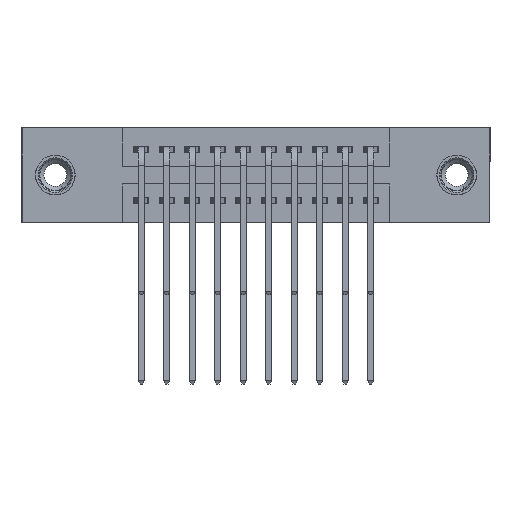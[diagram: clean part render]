
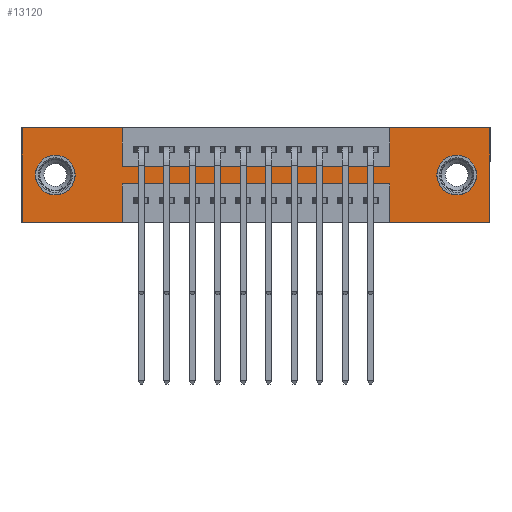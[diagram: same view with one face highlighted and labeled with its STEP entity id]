
A CAD part, front view. The second image highlights one B-rep face of the part: STEP entity #13120.
In plain terms, the highlighted planar face has unit normal (0, -1, 0).
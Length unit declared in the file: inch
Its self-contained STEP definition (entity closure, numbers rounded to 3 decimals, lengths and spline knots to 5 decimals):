
#68 = CARTESIAN_POINT ( 'NONE',  ( 0., 0., 0. ) ) ;
#136 = ORIENTED_EDGE ( 'NONE', *, *, #16094, .T. ) ;
#156 = VERTEX_POINT ( 'NONE', #68 ) ;
#206 = VECTOR ( 'NONE', #12975, 39.37008 ) ;
#285 = EDGE_CURVE ( 'NONE', #2101, #18559, #1158, .T. ) ;
#349 = CIRCLE ( 'NONE', #11111, 0.078 ) ;
#568 = CIRCLE ( 'NONE', #17081, 0.078 ) ;
#996 = CARTESIAN_POINT ( 'NONE',  ( 0.3925, 0., 0. ) ) ;
#1064 = EDGE_CURVE ( 'NONE', #9952, #18143, #1896, .T. ) ;
#1158 = LINE ( 'NONE', #2528, #15982 ) ;
#1196 = LINE ( 'NONE', #4455, #206 ) ;
#1268 = DIRECTION ( 'NONE',  ( 0., 0., 1. ) ) ;
#1285 = DIRECTION ( 'NONE',  ( 0., 0., -1. ) ) ;
#1363 = EDGE_LOOP ( 'NONE', ( #17937, #3118, #13664, #9716, #18570, #9848, #4302, #9397, #8794, #7609, #13158, #6612 ) ) ;
#1620 = FACE_BOUND ( 'NONE', #12168, .T. ) ;
#1694 = EDGE_CURVE ( 'NONE', #12277, #9224, #8646, .T. ) ;
#1896 = CIRCLE ( 'NONE', #10928, 0.078 ) ;
#2101 = VERTEX_POINT ( 'NONE', #16568 ) ;
#2160 = CARTESIAN_POINT ( 'NONE',  ( 0.3925, 0., -0.15 ) ) ;
#2228 = CARTESIAN_POINT ( 'NONE',  ( 0., 0., -0.37 ) ) ;
#2288 = DIRECTION ( 'NONE',  ( -1., 0., 0. ) ) ;
#2528 = CARTESIAN_POINT ( 'NONE',  ( 0.3925, 0., -0.22 ) ) ;
#2637 = EDGE_CURVE ( 'NONE', #7107, #156, #10333, .T. ) ;
#3118 = ORIENTED_EDGE ( 'NONE', *, *, #285, .F. ) ;
#3272 = AXIS2_PLACEMENT_3D ( 'NONE', #15878, #7675, #17248 ) ;
#3631 = VERTEX_POINT ( 'NONE', #15891 ) ;
#3795 = CARTESIAN_POINT ( 'NONE',  ( 1.4425, 0., -0.15 ) ) ;
#3831 = CARTESIAN_POINT ( 'NONE',  ( 1.705, 0., -0.185 ) ) ;
#4258 = VERTEX_POINT ( 'NONE', #6343 ) ;
#4271 = ORIENTED_EDGE ( 'NONE', *, *, #1064, .T. ) ;
#4302 = ORIENTED_EDGE ( 'NONE', *, *, #1694, .F. ) ;
#4362 = CARTESIAN_POINT ( 'NONE',  ( 1.4425, 0., -0.37 ) ) ;
#4455 = CARTESIAN_POINT ( 'NONE',  ( 0.3925, 0., -0.37 ) ) ;
#4488 = EDGE_CURVE ( 'NONE', #9224, #4258, #10752, .T. ) ;
#4766 = VECTOR ( 'NONE', #5490, 39.37008 ) ;
#4780 = VERTEX_POINT ( 'NONE', #8767 ) ;
#4819 = VERTEX_POINT ( 'NONE', #6131 ) ;
#4855 = PLANE ( 'NONE',  #9244 ) ;
#5021 = ORIENTED_EDGE ( 'NONE', *, *, #8070, .T. ) ;
#5112 = ORIENTED_EDGE ( 'NONE', *, *, #13055, .T. ) ;
#5213 = VERTEX_POINT ( 'NONE', #6851 ) ;
#5381 = VECTOR ( 'NONE', #12366, 39.37008 ) ;
#5400 = DIRECTION ( 'NONE',  ( 0., 0., -1. ) ) ;
#5413 = EDGE_CURVE ( 'NONE', #18559, #4780, #1196, .T. ) ;
#5490 = DIRECTION ( 'NONE',  ( 0., 0., 1. ) ) ;
#5999 = EDGE_LOOP ( 'NONE', ( #5021, #4271 ) ) ;
#6131 = CARTESIAN_POINT ( 'NONE',  ( 1.705, 0., -0.107 ) ) ;
#6231 = CIRCLE ( 'NONE', #3272, 0.078 ) ;
#6311 = VECTOR ( 'NONE', #13871, 39.37008 ) ;
#6343 = CARTESIAN_POINT ( 'NONE',  ( 1.835, 0., 0. ) ) ;
#6358 = DIRECTION ( 'NONE',  ( 0., 0., -1. ) ) ;
#6612 = ORIENTED_EDGE ( 'NONE', *, *, #12359, .F. ) ;
#6677 = VECTOR ( 'NONE', #1285, 39.37008 ) ;
#6706 = CARTESIAN_POINT ( 'NONE',  ( 1.705, 0., -0.263 ) ) ;
#6849 = CARTESIAN_POINT ( 'NONE',  ( 1.4425, 0., 0. ) ) ;
#6851 = CARTESIAN_POINT ( 'NONE',  ( 1.4425, 0., -0.37 ) ) ;
#6857 = EDGE_CURVE ( 'NONE', #5213, #2101, #11524, .T. ) ;
#6922 = CARTESIAN_POINT ( 'NONE',  ( 0., 0., -0.37 ) ) ;
#7107 = VERTEX_POINT ( 'NONE', #10768 ) ;
#7609 = ORIENTED_EDGE ( 'NONE', *, *, #13976, .F. ) ;
#7675 = DIRECTION ( 'NONE',  ( 0., 1., 0. ) ) ;
#7829 = VECTOR ( 'NONE', #18308, 39.37008 ) ;
#8070 = EDGE_CURVE ( 'NONE', #18143, #9952, #349, .T. ) ;
#8371 = CARTESIAN_POINT ( 'NONE',  ( 0.3925, 0., 0. ) ) ;
#8646 = LINE ( 'NONE', #13336, #4766 ) ;
#8759 = LINE ( 'NONE', #2160, #5381 ) ;
#8767 = CARTESIAN_POINT ( 'NONE',  ( 0.3925, 0., -0.37 ) ) ;
#8794 = ORIENTED_EDGE ( 'NONE', *, *, #18458, .F. ) ;
#9145 = FACE_OUTER_BOUND ( 'NONE', #1363, .T. ) ;
#9224 = VERTEX_POINT ( 'NONE', #6849 ) ;
#9244 = AXIS2_PLACEMENT_3D ( 'NONE', #13319, #14674, #6358 ) ;
#9397 = ORIENTED_EDGE ( 'NONE', *, *, #11238, .F. ) ;
#9634 = DIRECTION ( 'NONE',  ( 1., 0., 0. ) ) ;
#9641 = CARTESIAN_POINT ( 'NONE',  ( 0., 0., 0. ) ) ;
#9716 = ORIENTED_EDGE ( 'NONE', *, *, #13367, .F. ) ;
#9794 = VERTEX_POINT ( 'NONE', #6706 ) ;
#9814 = LINE ( 'NONE', #6922, #13033 ) ;
#9848 = ORIENTED_EDGE ( 'NONE', *, *, #4488, .F. ) ;
#9952 = VERTEX_POINT ( 'NONE', #16808 ) ;
#10135 = CARTESIAN_POINT ( 'NONE',  ( 0., 0., 0. ) ) ;
#10186 = DIRECTION ( 'NONE',  ( 0., 1., 0. ) ) ;
#10304 = VECTOR ( 'NONE', #16367, 39.37008 ) ;
#10333 = LINE ( 'NONE', #10135, #13141 ) ;
#10504 = CARTESIAN_POINT ( 'NONE',  ( 0.13, 0., -0.107 ) ) ;
#10752 = LINE ( 'NONE', #9641, #10304 ) ;
#10768 = CARTESIAN_POINT ( 'NONE',  ( 0., 0., -0.37 ) ) ;
#10928 = AXIS2_PLACEMENT_3D ( 'NONE', #18248, #17962, #14731 ) ;
#11111 = AXIS2_PLACEMENT_3D ( 'NONE', #18322, #10186, #1268 ) ;
#11238 = EDGE_CURVE ( 'NONE', #11624, #12277, #8759, .T. ) ;
#11524 = LINE ( 'NONE', #4362, #7829 ) ;
#11598 = CARTESIAN_POINT ( 'NONE',  ( 1.835, 0., 0. ) ) ;
#11624 = VERTEX_POINT ( 'NONE', #11793 ) ;
#11793 = CARTESIAN_POINT ( 'NONE',  ( 0.3925, 0., -0.15 ) ) ;
#12168 = EDGE_LOOP ( 'NONE', ( #5112, #136 ) ) ;
#12277 = VERTEX_POINT ( 'NONE', #3795 ) ;
#12359 = EDGE_CURVE ( 'NONE', #4780, #7107, #9814, .T. ) ;
#12366 = DIRECTION ( 'NONE',  ( 1., 0., 0. ) ) ;
#12414 = DIRECTION ( 'NONE',  ( -1., 0., 0. ) ) ;
#12554 = EDGE_CURVE ( 'NONE', #4258, #3631, #17653, .T. ) ;
#12583 = LINE ( 'NONE', #2228, #15708 ) ;
#12733 = CARTESIAN_POINT ( 'NONE',  ( 0.3925, 0., -0.22 ) ) ;
#12807 = FACE_BOUND ( 'NONE', #5999, .T. ) ;
#12975 = DIRECTION ( 'NONE',  ( 0., 0., -1. ) ) ;
#13033 = VECTOR ( 'NONE', #15196, 39.37008 ) ;
#13055 = EDGE_CURVE ( 'NONE', #4819, #9794, #6231, .T. ) ;
#13120 = ADVANCED_FACE ( 'NONE', ( #1620, #12807, #9145 ), #4855, .T. ) ;
#13136 = DIRECTION ( 'NONE',  ( 0., 0., 1. ) ) ;
#13141 = VECTOR ( 'NONE', #13136, 39.37008 ) ;
#13158 = ORIENTED_EDGE ( 'NONE', *, *, #2637, .F. ) ;
#13319 = CARTESIAN_POINT ( 'NONE',  ( 0., 0., -0.37 ) ) ;
#13336 = CARTESIAN_POINT ( 'NONE',  ( 1.4425, 0., 0. ) ) ;
#13367 = EDGE_CURVE ( 'NONE', #3631, #5213, #12583, .T. ) ;
#13664 = ORIENTED_EDGE ( 'NONE', *, *, #6857, .F. ) ;
#13802 = DIRECTION ( 'NONE',  ( 0., 1., 0. ) ) ;
#13871 = DIRECTION ( 'NONE',  ( 0., 0., -1. ) ) ;
#13976 = EDGE_CURVE ( 'NONE', #156, #18550, #16311, .T. ) ;
#14158 = LINE ( 'NONE', #8371, #6311 ) ;
#14674 = DIRECTION ( 'NONE',  ( 0., -1., 0. ) ) ;
#14731 = DIRECTION ( 'NONE',  ( 0., 0., 1. ) ) ;
#15196 = DIRECTION ( 'NONE',  ( -1., 0., 0. ) ) ;
#15708 = VECTOR ( 'NONE', #12414, 39.37008 ) ;
#15878 = CARTESIAN_POINT ( 'NONE',  ( 1.705, 0., -0.185 ) ) ;
#15891 = CARTESIAN_POINT ( 'NONE',  ( 1.835, 0., -0.37 ) ) ;
#15982 = VECTOR ( 'NONE', #2288, 39.37008 ) ;
#16094 = EDGE_CURVE ( 'NONE', #9794, #4819, #568, .T. ) ;
#16311 = LINE ( 'NONE', #17748, #16744 ) ;
#16367 = DIRECTION ( 'NONE',  ( 1., 0., 0. ) ) ;
#16568 = CARTESIAN_POINT ( 'NONE',  ( 1.4425, 0., -0.22 ) ) ;
#16744 = VECTOR ( 'NONE', #9634, 39.37008 ) ;
#16808 = CARTESIAN_POINT ( 'NONE',  ( 0.13, 0., -0.263 ) ) ;
#17081 = AXIS2_PLACEMENT_3D ( 'NONE', #3831, #13802, #5400 ) ;
#17248 = DIRECTION ( 'NONE',  ( 0., 0., -1. ) ) ;
#17653 = LINE ( 'NONE', #11598, #6677 ) ;
#17748 = CARTESIAN_POINT ( 'NONE',  ( 0., 0., 0. ) ) ;
#17937 = ORIENTED_EDGE ( 'NONE', *, *, #5413, .F. ) ;
#17962 = DIRECTION ( 'NONE',  ( 0., 1., 0. ) ) ;
#18143 = VERTEX_POINT ( 'NONE', #10504 ) ;
#18248 = CARTESIAN_POINT ( 'NONE',  ( 0.13, 0., -0.185 ) ) ;
#18308 = DIRECTION ( 'NONE',  ( 0., 0., 1. ) ) ;
#18322 = CARTESIAN_POINT ( 'NONE',  ( 0.13, 0., -0.185 ) ) ;
#18458 = EDGE_CURVE ( 'NONE', #18550, #11624, #14158, .T. ) ;
#18550 = VERTEX_POINT ( 'NONE', #996 ) ;
#18559 = VERTEX_POINT ( 'NONE', #12733 ) ;
#18570 = ORIENTED_EDGE ( 'NONE', *, *, #12554, .F. ) ;
